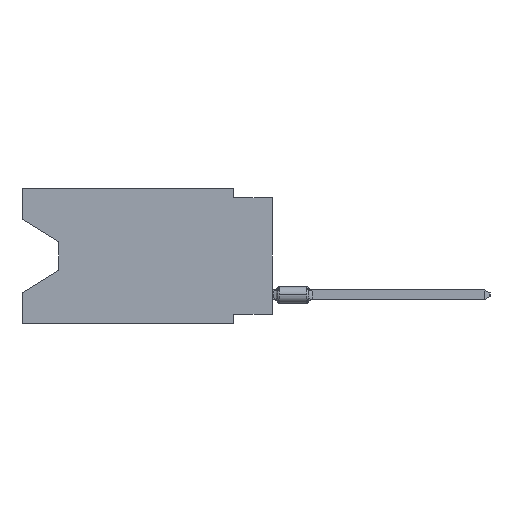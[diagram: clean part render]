
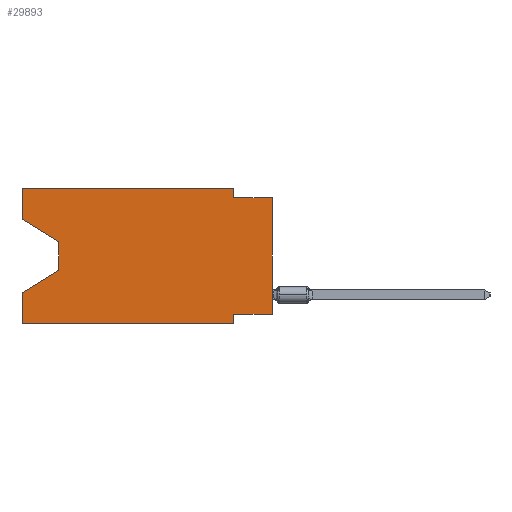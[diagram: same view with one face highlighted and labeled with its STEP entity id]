
A CAD part, left-side view. The second image highlights one B-rep face of the part: STEP entity #29893.
In plain terms, the highlighted planar face has unit normal (-1, 0, 0).
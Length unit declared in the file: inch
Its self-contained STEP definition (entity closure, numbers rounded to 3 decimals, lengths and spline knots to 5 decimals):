
#691 = DIRECTION ( 'NONE',  ( 0., 0., -1. ) ) ;
#741 = EDGE_CURVE ( 'NONE', #15696, #22835, #35294, .T. ) ;
#1053 = ORIENTED_EDGE ( 'NONE', *, *, #33774, .F. ) ;
#1794 = CARTESIAN_POINT ( 'NONE',  ( 0., 0., -0.325 ) ) ;
#1946 = CARTESIAN_POINT ( 'NONE',  ( 0., 0.645, -0.08025 ) ) ;
#1959 = LINE ( 'NONE', #29518, #34440 ) ;
#3204 = CARTESIAN_POINT ( 'NONE',  ( 0., 0.645, 0. ) ) ;
#4103 = EDGE_CURVE ( 'NONE', #12892, #20458, #27537, .T. ) ;
#4662 = LINE ( 'NONE', #26188, #12953 ) ;
#6282 = CARTESIAN_POINT ( 'NONE',  ( 0., 0.645, 0. ) ) ;
#6524 = VECTOR ( 'NONE', #11153, 39.37008 ) ;
#6707 = CARTESIAN_POINT ( 'NONE',  ( 0., 0.645, -0.35 ) ) ;
#6787 = ORIENTED_EDGE ( 'NONE', *, *, #30083, .F. ) ;
#6914 = ORIENTED_EDGE ( 'NONE', *, *, #8465, .F. ) ;
#7386 = EDGE_CURVE ( 'NONE', #22835, #37748, #21114, .T. ) ;
#7623 = CARTESIAN_POINT ( 'NONE',  ( 0., 0.645, 0. ) ) ;
#7683 = ORIENTED_EDGE ( 'NONE', *, *, #35674, .T. ) ;
#7755 = ORIENTED_EDGE ( 'NONE', *, *, #21390, .T. ) ;
#8142 = LINE ( 'NONE', #29485, #10886 ) ;
#8218 = LINE ( 'NONE', #32966, #28470 ) ;
#8465 = EDGE_CURVE ( 'NONE', #15121, #36301, #22816, .T. ) ;
#8499 = LINE ( 'NONE', #13941, #24363 ) ;
#8896 = DIRECTION ( 'NONE',  ( 0., -1., 0. ) ) ;
#9280 = ORIENTED_EDGE ( 'NONE', *, *, #7386, .F. ) ;
#9300 = PLANE ( 'NONE',  #18827 ) ;
#9966 = VECTOR ( 'NONE', #35398, 39.37008 ) ;
#10321 = ORIENTED_EDGE ( 'NONE', *, *, #16449, .T. ) ;
#10886 = VECTOR ( 'NONE', #22857, 39.37008 ) ;
#11153 = DIRECTION ( 'NONE',  ( 0., 0., 1. ) ) ;
#11293 = ORIENTED_EDGE ( 'NONE', *, *, #4103, .T. ) ;
#11299 = EDGE_LOOP ( 'NONE', ( #10321, #16843, #11293, #1053, #7755, #6914, #26790, #7683, #6787, #9280, #36137, #20901 ) ) ;
#12247 = CARTESIAN_POINT ( 'NONE',  ( 0., 0.55, -0.212 ) ) ;
#12892 = VERTEX_POINT ( 'NONE', #38235 ) ;
#12953 = VECTOR ( 'NONE', #38463, 39.37008 ) ;
#13228 = CARTESIAN_POINT ( 'NONE',  ( 0., 0.645, -0.26975 ) ) ;
#13592 = CARTESIAN_POINT ( 'NONE',  ( 0., 0.1, -0.325 ) ) ;
#13941 = CARTESIAN_POINT ( 'NONE',  ( 0., 0.645, 0. ) ) ;
#14752 = LINE ( 'NONE', #20396, #6524 ) ;
#15121 = VERTEX_POINT ( 'NONE', #13592 ) ;
#15370 = VERTEX_POINT ( 'NONE', #24045 ) ;
#15696 = VERTEX_POINT ( 'NONE', #3204 ) ;
#16449 = EDGE_CURVE ( 'NONE', #31046, #15370, #8142, .T. ) ;
#16588 = VECTOR ( 'NONE', #39234, 39.37008 ) ;
#16690 = DIRECTION ( 'NONE',  ( 0., 0., -1. ) ) ;
#16843 = ORIENTED_EDGE ( 'NONE', *, *, #36447, .T. ) ;
#17038 = DIRECTION ( 'NONE',  ( 0., -1., 0. ) ) ;
#17845 = EDGE_CURVE ( 'NONE', #31046, #15696, #8499, .T. ) ;
#18827 = AXIS2_PLACEMENT_3D ( 'NONE', #6282, #36870, #16690 ) ;
#20396 = CARTESIAN_POINT ( 'NONE',  ( 0., 0., 0. ) ) ;
#20458 = VERTEX_POINT ( 'NONE', #13228 ) ;
#20901 = ORIENTED_EDGE ( 'NONE', *, *, #17845, .F. ) ;
#20985 = VECTOR ( 'NONE', #36797, 39.37008 ) ;
#21114 = LINE ( 'NONE', #36600, #16588 ) ;
#21390 = EDGE_CURVE ( 'NONE', #39238, #36301, #1959, .T. ) ;
#21576 = CARTESIAN_POINT ( 'NONE',  ( 0., 0.1, -0.35 ) ) ;
#22210 = CARTESIAN_POINT ( 'NONE',  ( 0., 0.1, -0.35 ) ) ;
#22790 = CARTESIAN_POINT ( 'NONE',  ( 0., 0., -0.325 ) ) ;
#22816 = LINE ( 'NONE', #22210, #28752 ) ;
#22835 = VERTEX_POINT ( 'NONE', #29263 ) ;
#22857 = DIRECTION ( 'NONE',  ( 0., -0.855, -0.519 ) ) ;
#24045 = CARTESIAN_POINT ( 'NONE',  ( 0., 0.55, -0.138 ) ) ;
#24363 = VECTOR ( 'NONE', #33653, 39.37008 ) ;
#24369 = CARTESIAN_POINT ( 'NONE',  ( 0., 0.1, -0.025 ) ) ;
#25343 = VECTOR ( 'NONE', #8896, 39.37008 ) ;
#26188 = CARTESIAN_POINT ( 'NONE',  ( 0., 0.55, -0.138 ) ) ;
#26629 = VERTEX_POINT ( 'NONE', #1794 ) ;
#26790 = ORIENTED_EDGE ( 'NONE', *, *, #37591, .F. ) ;
#27537 = LINE ( 'NONE', #12247, #20985 ) ;
#28470 = VECTOR ( 'NONE', #35988, 39.37008 ) ;
#28752 = VECTOR ( 'NONE', #691, 39.37008 ) ;
#29247 = CARTESIAN_POINT ( 'NONE',  ( 0., 0.645, 0. ) ) ;
#29263 = CARTESIAN_POINT ( 'NONE',  ( 0., 0.1, 0. ) ) ;
#29485 = CARTESIAN_POINT ( 'NONE',  ( 0., 0.645, -0.08025 ) ) ;
#29518 = CARTESIAN_POINT ( 'NONE',  ( 0., 0.645, -0.35 ) ) ;
#29893 = ADVANCED_FACE ( 'NONE', ( #34257 ), #9300, .F. ) ;
#30083 = EDGE_CURVE ( 'NONE', #37748, #33221, #8218, .T. ) ;
#31046 = VERTEX_POINT ( 'NONE', #1946 ) ;
#32430 = LINE ( 'NONE', #22790, #39382 ) ;
#32766 = LINE ( 'NONE', #7623, #9966 ) ;
#32966 = CARTESIAN_POINT ( 'NONE',  ( 0., 0., -0.025 ) ) ;
#33221 = VERTEX_POINT ( 'NONE', #34296 ) ;
#33653 = DIRECTION ( 'NONE',  ( 0., 0., 1. ) ) ;
#33774 = EDGE_CURVE ( 'NONE', #39238, #20458, #32766, .T. ) ;
#34257 = FACE_OUTER_BOUND ( 'NONE', #11299, .T. ) ;
#34296 = CARTESIAN_POINT ( 'NONE',  ( 0., 0., -0.025 ) ) ;
#34440 = VECTOR ( 'NONE', #17038, 39.37008 ) ;
#35258 = DIRECTION ( 'NONE',  ( 0., 1., 0. ) ) ;
#35294 = LINE ( 'NONE', #29247, #25343 ) ;
#35398 = DIRECTION ( 'NONE',  ( 0., 0., 1. ) ) ;
#35674 = EDGE_CURVE ( 'NONE', #26629, #33221, #14752, .T. ) ;
#35988 = DIRECTION ( 'NONE',  ( 0., -1., 0. ) ) ;
#36137 = ORIENTED_EDGE ( 'NONE', *, *, #741, .F. ) ;
#36301 = VERTEX_POINT ( 'NONE', #21576 ) ;
#36447 = EDGE_CURVE ( 'NONE', #15370, #12892, #4662, .T. ) ;
#36600 = CARTESIAN_POINT ( 'NONE',  ( 0., 0.1, 0. ) ) ;
#36797 = DIRECTION ( 'NONE',  ( 0., 0.855, -0.519 ) ) ;
#36870 = DIRECTION ( 'NONE',  ( 1., 0., 0. ) ) ;
#37591 = EDGE_CURVE ( 'NONE', #26629, #15121, #32430, .T. ) ;
#37748 = VERTEX_POINT ( 'NONE', #24369 ) ;
#38235 = CARTESIAN_POINT ( 'NONE',  ( 0., 0.55, -0.212 ) ) ;
#38463 = DIRECTION ( 'NONE',  ( 0., 0., -1. ) ) ;
#39234 = DIRECTION ( 'NONE',  ( 0., 0., -1. ) ) ;
#39238 = VERTEX_POINT ( 'NONE', #6707 ) ;
#39382 = VECTOR ( 'NONE', #35258, 39.37008 ) ;
